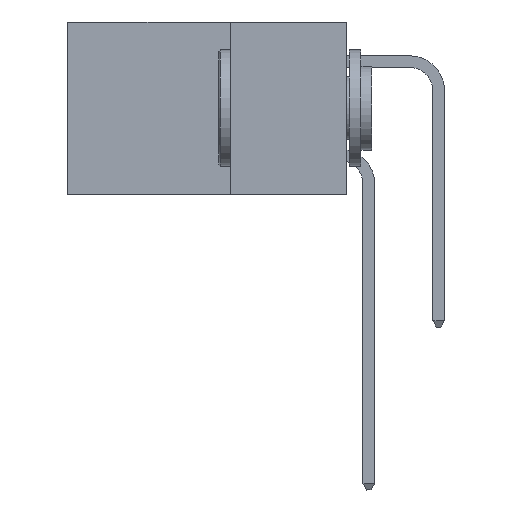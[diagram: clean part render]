
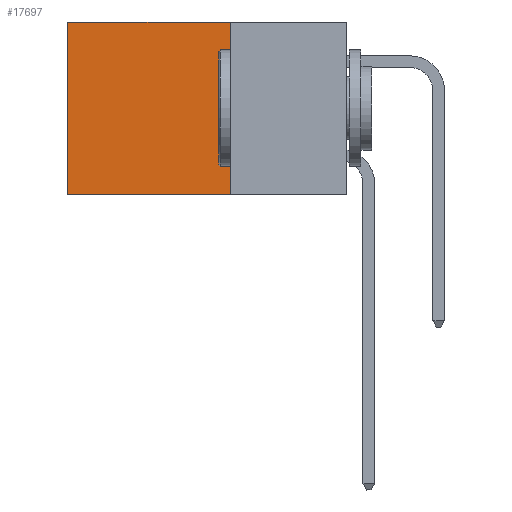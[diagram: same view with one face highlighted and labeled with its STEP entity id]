
A CAD part, left-side view. The second image highlights one B-rep face of the part: STEP entity #17697.
In plain terms, the highlighted planar face has unit normal (-1, 0, 0).
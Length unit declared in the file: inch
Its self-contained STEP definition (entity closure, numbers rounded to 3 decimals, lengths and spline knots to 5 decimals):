
#563 = LINE ( 'NONE', #13538, #17412 ) ;
#957 = FACE_OUTER_BOUND ( 'NONE', #7094, .T. ) ;
#1408 = EDGE_CURVE ( 'NONE', #8082, #16629, #2531, .T. ) ;
#1409 = ORIENTED_EDGE ( 'NONE', *, *, #9894, .F. ) ;
#2531 = LINE ( 'NONE', #15353, #6379 ) ;
#3013 = CARTESIAN_POINT ( 'NONE',  ( 0.2875, 0.25, -0.37 ) ) ;
#3107 = DIRECTION ( 'NONE',  ( 0., 0., -1. ) ) ;
#4254 = CARTESIAN_POINT ( 'NONE',  ( 0.2875, 0.25, 0. ) ) ;
#4635 = DIRECTION ( 'NONE',  ( 0., 1., 0. ) ) ;
#4667 = VECTOR ( 'NONE', #4635, 39.37008 ) ;
#6141 = CARTESIAN_POINT ( 'NONE',  ( 0.2875, 0.6, 0. ) ) ;
#6223 = EDGE_CURVE ( 'NONE', #12160, #16629, #9001, .T. ) ;
#6379 = VECTOR ( 'NONE', #6636, 39.37008 ) ;
#6636 = DIRECTION ( 'NONE',  ( 0., 0., -1. ) ) ;
#6832 = VECTOR ( 'NONE', #8823, 39.37008 ) ;
#7094 = EDGE_LOOP ( 'NONE', ( #12049, #12671, #1409, #9720 ) ) ;
#7145 = DIRECTION ( 'NONE',  ( 0., 0., -1. ) ) ;
#8082 = VERTEX_POINT ( 'NONE', #6141 ) ;
#8823 = DIRECTION ( 'NONE',  ( 0., 1., 0. ) ) ;
#9001 = LINE ( 'NONE', #9273, #4667 ) ;
#9273 = CARTESIAN_POINT ( 'NONE',  ( 0.2875, 0.25, -0.37 ) ) ;
#9575 = PLANE ( 'NONE',  #11913 ) ;
#9720 = ORIENTED_EDGE ( 'NONE', *, *, #17146, .T. ) ;
#9894 = EDGE_CURVE ( 'NONE', #17502, #12160, #563, .T. ) ;
#11913 = AXIS2_PLACEMENT_3D ( 'NONE', #20234, #12759, #3107 ) ;
#12049 = ORIENTED_EDGE ( 'NONE', *, *, #1408, .T. ) ;
#12053 = CARTESIAN_POINT ( 'NONE',  ( 0.2875, 0.6, -0.37 ) ) ;
#12160 = VERTEX_POINT ( 'NONE', #3013 ) ;
#12671 = ORIENTED_EDGE ( 'NONE', *, *, #6223, .F. ) ;
#12759 = DIRECTION ( 'NONE',  ( 1., 0., 0. ) ) ;
#13538 = CARTESIAN_POINT ( 'NONE',  ( 0.2875, 0.25, 0. ) ) ;
#13569 = CARTESIAN_POINT ( 'NONE',  ( 0.2875, 0.25, 0. ) ) ;
#15353 = CARTESIAN_POINT ( 'NONE',  ( 0.2875, 0.6, 0. ) ) ;
#16629 = VERTEX_POINT ( 'NONE', #12053 ) ;
#17146 = EDGE_CURVE ( 'NONE', #17502, #8082, #19196, .T. ) ;
#17412 = VECTOR ( 'NONE', #7145, 39.37008 ) ;
#17502 = VERTEX_POINT ( 'NONE', #4254 ) ;
#17697 = ADVANCED_FACE ( 'NONE', ( #957 ), #9575, .F. ) ;
#19196 = LINE ( 'NONE', #13569, #6832 ) ;
#20234 = CARTESIAN_POINT ( 'NONE',  ( 0.2875, 0.25, 0. ) ) ;
